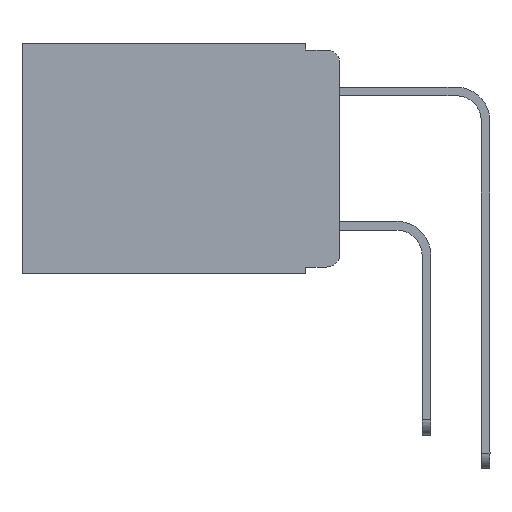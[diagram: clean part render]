
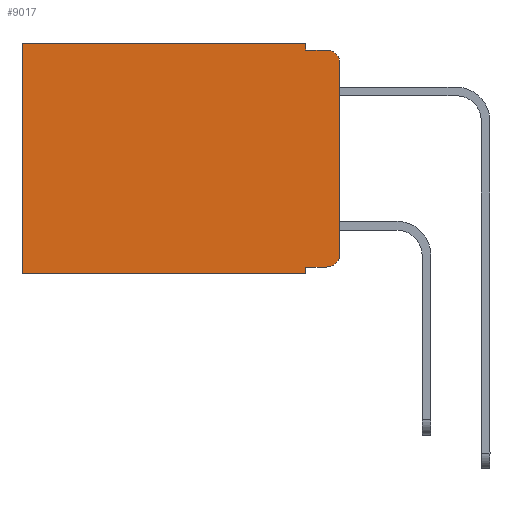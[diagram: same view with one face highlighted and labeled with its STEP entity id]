
A CAD part, left-side view. The second image highlights one B-rep face of the part: STEP entity #9017.
In plain terms, the highlighted planar face has unit normal (-1, 0, 0).
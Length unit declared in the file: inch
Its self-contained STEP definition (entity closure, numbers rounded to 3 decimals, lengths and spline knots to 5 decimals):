
#53 = DIRECTION ( 'NONE',  ( 0., -1., 0. ) ) ;
#127 = VERTEX_POINT ( 'NONE', #2749 ) ;
#251 = VECTOR ( 'NONE', #7604, 39.37008 ) ;
#325 = EDGE_CURVE ( 'NONE', #7385, #11708, #8896, .T. ) ;
#393 = VECTOR ( 'NONE', #6445, 39.37008 ) ;
#505 = LINE ( 'NONE', #9237, #4317 ) ;
#539 = EDGE_CURVE ( 'NONE', #9304, #127, #905, .T. ) ;
#839 = EDGE_CURVE ( 'NONE', #1038, #9573, #505, .T. ) ;
#867 = ORIENTED_EDGE ( 'NONE', *, *, #11424, .F. ) ;
#876 = LINE ( 'NONE', #4745, #12109 ) ;
#895 = ORIENTED_EDGE ( 'NONE', *, *, #4339, .F. ) ;
#905 = LINE ( 'NONE', #8426, #251 ) ;
#976 = PLANE ( 'NONE',  #2392 ) ;
#1038 = VERTEX_POINT ( 'NONE', #8754 ) ;
#1264 = CARTESIAN_POINT ( 'NONE',  ( 0.298, 0.473, 0. ) ) ;
#1302 = VERTEX_POINT ( 'NONE', #10304 ) ;
#1793 = CIRCLE ( 'NONE', #6835, 0.02 ) ;
#2036 = CARTESIAN_POINT ( 'NONE',  ( 0.298, 0.473, 0. ) ) ;
#2147 = DIRECTION ( 'NONE',  ( -1., 0., 0. ) ) ;
#2282 = CARTESIAN_POINT ( 'NONE',  ( 0.298, 0.02, -0.313 ) ) ;
#2392 = AXIS2_PLACEMENT_3D ( 'NONE', #10765, #12405, #9703 ) ;
#2429 = EDGE_CURVE ( 'NONE', #3691, #9573, #6834, .T. ) ;
#2472 = LINE ( 'NONE', #5491, #12192 ) ;
#2513 = VECTOR ( 'NONE', #7888, 39.37008 ) ;
#2749 = CARTESIAN_POINT ( 'NONE',  ( 0.298, 0.02, -0.333 ) ) ;
#3235 = VERTEX_POINT ( 'NONE', #4723 ) ;
#3691 = VERTEX_POINT ( 'NONE', #1264 ) ;
#4053 = CARTESIAN_POINT ( 'NONE',  ( 0.298, 0.051, -0.01 ) ) ;
#4285 = EDGE_CURVE ( 'NONE', #10958, #3691, #11232, .T. ) ;
#4317 = VECTOR ( 'NONE', #11075, 39.37008 ) ;
#4339 = EDGE_CURVE ( 'NONE', #3235, #1302, #2472, .T. ) ;
#4416 = DIRECTION ( 'NONE',  ( 0., 1., 0. ) ) ;
#4617 = LINE ( 'NONE', #9346, #393 ) ;
#4723 = CARTESIAN_POINT ( 'NONE',  ( 0.298, 0., -0.03 ) ) ;
#4745 = CARTESIAN_POINT ( 'NONE',  ( 0.298, 0.051, 0. ) ) ;
#5459 = ORIENTED_EDGE ( 'NONE', *, *, #11576, .T. ) ;
#5491 = CARTESIAN_POINT ( 'NONE',  ( 0.298, 0., 0. ) ) ;
#5737 = CARTESIAN_POINT ( 'NONE',  ( 0.298, 0.02, -0.03 ) ) ;
#6445 = DIRECTION ( 'NONE',  ( 0., 0., -1. ) ) ;
#6834 = LINE ( 'NONE', #2036, #2513 ) ;
#6835 = AXIS2_PLACEMENT_3D ( 'NONE', #2282, #2147, #10933 ) ;
#6844 = VECTOR ( 'NONE', #53, 39.37008 ) ;
#6874 = CARTESIAN_POINT ( 'NONE',  ( 0.298, 0.02, -0.01 ) ) ;
#7385 = VERTEX_POINT ( 'NONE', #4053 ) ;
#7604 = DIRECTION ( 'NONE',  ( 0., -1., 0. ) ) ;
#7645 = ORIENTED_EDGE ( 'NONE', *, *, #839, .F. ) ;
#7684 = ORIENTED_EDGE ( 'NONE', *, *, #10001, .T. ) ;
#7713 = ORIENTED_EDGE ( 'NONE', *, *, #4285, .T. ) ;
#7728 = CARTESIAN_POINT ( 'NONE',  ( 0.298, 0.051, 0. ) ) ;
#7743 = DIRECTION ( 'NONE',  ( 0., 0., -1. ) ) ;
#7794 = ORIENTED_EDGE ( 'NONE', *, *, #325, .F. ) ;
#7888 = DIRECTION ( 'NONE',  ( 0., 0., -1. ) ) ;
#7892 = CARTESIAN_POINT ( 'NONE',  ( 0.298, 0.473, -0.343 ) ) ;
#8044 = AXIS2_PLACEMENT_3D ( 'NONE', #5737, #11491, #10501 ) ;
#8077 = ORIENTED_EDGE ( 'NONE', *, *, #539, .T. ) ;
#8124 = DIRECTION ( 'NONE',  ( 0., 0., -1. ) ) ;
#8426 = CARTESIAN_POINT ( 'NONE',  ( 0.298, 0.051, -0.333 ) ) ;
#8754 = CARTESIAN_POINT ( 'NONE',  ( 0.298, 0.051, -0.343 ) ) ;
#8896 = LINE ( 'NONE', #9927, #6844 ) ;
#9017 = ADVANCED_FACE ( 'NONE', ( #9828 ), #976, .F. ) ;
#9101 = ORIENTED_EDGE ( 'NONE', *, *, #2429, .T. ) ;
#9237 = CARTESIAN_POINT ( 'NONE',  ( 0.298, 0., -0.343 ) ) ;
#9304 = VERTEX_POINT ( 'NONE', #10285 ) ;
#9346 = CARTESIAN_POINT ( 'NONE',  ( 0.298, 0.051, 0. ) ) ;
#9540 = EDGE_LOOP ( 'NONE', ( #895, #5459, #7794, #867, #7713, #9101, #7645, #10328, #8077, #7684 ) ) ;
#9573 = VERTEX_POINT ( 'NONE', #7892 ) ;
#9703 = DIRECTION ( 'NONE',  ( 0., 0., -1. ) ) ;
#9828 = FACE_OUTER_BOUND ( 'NONE', #9540, .T. ) ;
#9927 = CARTESIAN_POINT ( 'NONE',  ( 0.298, 0.051, -0.01 ) ) ;
#10001 = EDGE_CURVE ( 'NONE', #127, #1302, #1793, .T. ) ;
#10285 = CARTESIAN_POINT ( 'NONE',  ( 0.298, 0.051, -0.333 ) ) ;
#10304 = CARTESIAN_POINT ( 'NONE',  ( 0.298, 0., -0.313 ) ) ;
#10328 = ORIENTED_EDGE ( 'NONE', *, *, #11622, .F. ) ;
#10501 = DIRECTION ( 'NONE',  ( 0., 0., -1. ) ) ;
#10765 = CARTESIAN_POINT ( 'NONE',  ( 0.298, 0., 0. ) ) ;
#10933 = DIRECTION ( 'NONE',  ( 0., 0., -1. ) ) ;
#10958 = VERTEX_POINT ( 'NONE', #7728 ) ;
#11075 = DIRECTION ( 'NONE',  ( 0., 1., 0. ) ) ;
#11232 = LINE ( 'NONE', #12121, #11999 ) ;
#11424 = EDGE_CURVE ( 'NONE', #10958, #7385, #4617, .T. ) ;
#11491 = DIRECTION ( 'NONE',  ( -1., 0., 0. ) ) ;
#11576 = EDGE_CURVE ( 'NONE', #3235, #11708, #11696, .T. ) ;
#11622 = EDGE_CURVE ( 'NONE', #9304, #1038, #876, .T. ) ;
#11696 = CIRCLE ( 'NONE', #8044, 0.02 ) ;
#11708 = VERTEX_POINT ( 'NONE', #6874 ) ;
#11999 = VECTOR ( 'NONE', #4416, 39.37008 ) ;
#12109 = VECTOR ( 'NONE', #7743, 39.37008 ) ;
#12121 = CARTESIAN_POINT ( 'NONE',  ( 0.298, 0., 0. ) ) ;
#12192 = VECTOR ( 'NONE', #8124, 39.37008 ) ;
#12405 = DIRECTION ( 'NONE',  ( 1., 0., 0. ) ) ;
